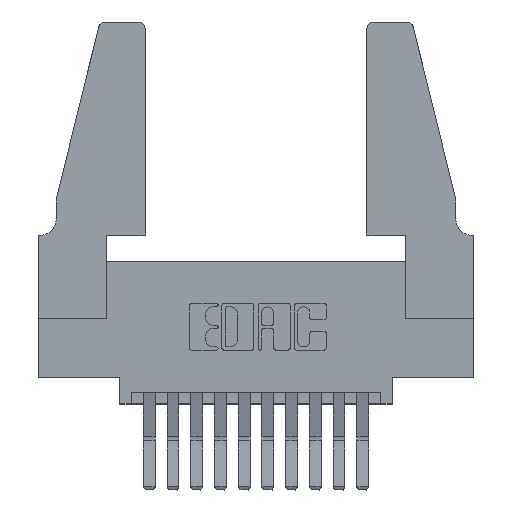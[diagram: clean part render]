
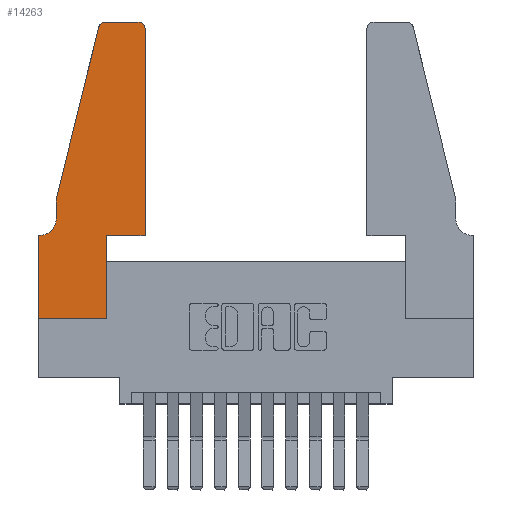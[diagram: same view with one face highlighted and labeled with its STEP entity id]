
A CAD part, top view. The second image highlights one B-rep face of the part: STEP entity #14263.
In plain terms, the highlighted planar face has unit normal (0, 0, 1).
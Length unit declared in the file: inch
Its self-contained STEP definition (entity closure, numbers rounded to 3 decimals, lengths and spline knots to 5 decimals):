
#20 = ORIENTED_EDGE ( 'NONE', *, *, #10793, .T. ) ;
#134 = VERTEX_POINT ( 'NONE', #2024 ) ;
#516 = CARTESIAN_POINT ( 'NONE',  ( 0.0755, 0.5, 0.37 ) ) ;
#620 = VERTEX_POINT ( 'NONE', #7448 ) ;
#683 = DIRECTION ( 'NONE',  ( 1., 0., 0. ) ) ;
#951 = CARTESIAN_POINT ( 'NONE',  ( 0.0755, 0.5, 0.37 ) ) ;
#965 = CARTESIAN_POINT ( 'NONE',  ( 0.4205, 1.22, 0.37 ) ) ;
#1316 = CARTESIAN_POINT ( 'NONE',  ( 0.0755, 0.5, 0.37 ) ) ;
#1519 = CARTESIAN_POINT ( 'NONE',  ( 0.2865, 0.35, 0.37 ) ) ;
#1893 = ORIENTED_EDGE ( 'NONE', *, *, #11716, .T. ) ;
#1920 = VECTOR ( 'NONE', #12752, 39.37008 ) ;
#2024 = CARTESIAN_POINT ( 'NONE',  ( 0., 0.35, 0.37 ) ) ;
#2279 = LINE ( 'NONE', #14541, #7880 ) ;
#2289 = DIRECTION ( 'NONE',  ( 1., 0., 0. ) ) ;
#2481 = CARTESIAN_POINT ( 'NONE',  ( 0.4205, 1.25, 0.37 ) ) ;
#2592 = DIRECTION ( 'NONE',  ( 0., -1., 0. ) ) ;
#2875 = EDGE_CURVE ( 'NONE', #134, #13438, #4953, .T. ) ;
#2930 = CIRCLE ( 'NONE', #3159, 0.03 ) ;
#3159 = AXIS2_PLACEMENT_3D ( 'NONE', #14060, #7624, #683 ) ;
#3321 = DIRECTION ( 'NONE',  ( 1., 0., 0. ) ) ;
#3361 = VERTEX_POINT ( 'NONE', #516 ) ;
#3426 = ORIENTED_EDGE ( 'NONE', *, *, #2875, .T. ) ;
#3492 = VECTOR ( 'NONE', #9399, 39.37008 ) ;
#3600 = VECTOR ( 'NONE', #2592, 39.37008 ) ;
#3761 = CARTESIAN_POINT ( 'NONE',  ( 0.4505, 0.35, 0.37 ) ) ;
#3775 = EDGE_CURVE ( 'NONE', #9336, #134, #2279, .T. ) ;
#3909 = CARTESIAN_POINT ( 'NONE',  ( 0.284, 1.25, 0.37 ) ) ;
#3928 = DIRECTION ( 'NONE',  ( -1., 0., 0. ) ) ;
#4141 = EDGE_CURVE ( 'NONE', #9167, #12550, #11786, .T. ) ;
#4200 = CARTESIAN_POINT ( 'NONE',  ( 0.4505, 1.22, 0.37 ) ) ;
#4295 = VECTOR ( 'NONE', #12698, 39.37008 ) ;
#4298 = EDGE_LOOP ( 'NONE', ( #11027, #5619, #14450, #20, #6785, #9504, #3426, #1893, #11402, #11693, #12188, #13279 ) ) ;
#4350 = VERTEX_POINT ( 'NONE', #4902 ) ;
#4546 = LINE ( 'NONE', #14178, #10050 ) ;
#4716 = EDGE_CURVE ( 'NONE', #6889, #4350, #4546, .T. ) ;
#4836 = DIRECTION ( 'NONE',  ( 0., 1., 0. ) ) ;
#4902 = CARTESIAN_POINT ( 'NONE',  ( 0.4505, 0.35, 0.37 ) ) ;
#4953 = LINE ( 'NONE', #8320, #1920 ) ;
#4991 = EDGE_CURVE ( 'NONE', #4350, #9167, #13086, .T. ) ;
#5003 = FACE_OUTER_BOUND ( 'NONE', #4298, .T. ) ;
#5048 = CARTESIAN_POINT ( 'NONE',  ( 0.2605, 1.25, 0.37 ) ) ;
#5599 = DIRECTION ( 'NONE',  ( -0.239, -0.971, 0. ) ) ;
#5619 = ORIENTED_EDGE ( 'NONE', *, *, #12937, .T. ) ;
#5859 = AXIS2_PLACEMENT_3D ( 'NONE', #965, #8966, #2289 ) ;
#6096 = DIRECTION ( 'NONE',  ( 0., 0., -1. ) ) ;
#6759 = AXIS2_PLACEMENT_3D ( 'NONE', #12670, #6096, #13705 ) ;
#6785 = ORIENTED_EDGE ( 'NONE', *, *, #11508, .T. ) ;
#6889 = VERTEX_POINT ( 'NONE', #13394 ) ;
#7047 = CARTESIAN_POINT ( 'NONE',  ( 0.25487, 1.22718, 0.37 ) ) ;
#7448 = CARTESIAN_POINT ( 'NONE',  ( 0.0755, 0.42, 0.37 ) ) ;
#7624 = DIRECTION ( 'NONE',  ( 0., 0., 1. ) ) ;
#7803 = VECTOR ( 'NONE', #5599, 39.37008 ) ;
#7880 = VECTOR ( 'NONE', #3928, 39.37008 ) ;
#8271 = CIRCLE ( 'NONE', #6759, 0.07 ) ;
#8320 = CARTESIAN_POINT ( 'NONE',  ( 0., 0., 0.37 ) ) ;
#8389 = EDGE_CURVE ( 'NONE', #8887, #6889, #9370, .T. ) ;
#8843 = PLANE ( 'NONE',  #11649 ) ;
#8887 = VERTEX_POINT ( 'NONE', #13555 ) ;
#8966 = DIRECTION ( 'NONE',  ( 0., 0., 1. ) ) ;
#8980 = VERTEX_POINT ( 'NONE', #3909 ) ;
#9167 = VERTEX_POINT ( 'NONE', #4200 ) ;
#9336 = VERTEX_POINT ( 'NONE', #13273 ) ;
#9370 = LINE ( 'NONE', #1519, #3492 ) ;
#9399 = DIRECTION ( 'NONE',  ( 0., 1., 0. ) ) ;
#9504 = ORIENTED_EDGE ( 'NONE', *, *, #3775, .T. ) ;
#9874 = CARTESIAN_POINT ( 'NONE',  ( 0., 0., 0.37 ) ) ;
#9928 = DIRECTION ( 'NONE',  ( 0., 0., 1. ) ) ;
#10050 = VECTOR ( 'NONE', #13141, 39.37008 ) ;
#10300 = EDGE_CURVE ( 'NONE', #12550, #8980, #12696, .T. ) ;
#10358 = LINE ( 'NONE', #951, #7803 ) ;
#10793 = EDGE_CURVE ( 'NONE', #3361, #620, #12368, .T. ) ;
#10971 = CARTESIAN_POINT ( 'NONE',  ( 0., 0.35, 0.37 ) ) ;
#11027 = ORIENTED_EDGE ( 'NONE', *, *, #10300, .T. ) ;
#11297 = VECTOR ( 'NONE', #13169, 39.37008 ) ;
#11402 = ORIENTED_EDGE ( 'NONE', *, *, #8389, .T. ) ;
#11439 = VERTEX_POINT ( 'NONE', #7047 ) ;
#11508 = EDGE_CURVE ( 'NONE', #620, #9336, #8271, .T. ) ;
#11649 = AXIS2_PLACEMENT_3D ( 'NONE', #10971, #9928, #3321 ) ;
#11693 = ORIENTED_EDGE ( 'NONE', *, *, #4716, .T. ) ;
#11716 = EDGE_CURVE ( 'NONE', #13438, #8887, #14117, .T. ) ;
#11786 = CIRCLE ( 'NONE', #5859, 0.03 ) ;
#12096 = VECTOR ( 'NONE', #4836, 39.37008 ) ;
#12188 = ORIENTED_EDGE ( 'NONE', *, *, #4991, .T. ) ;
#12368 = LINE ( 'NONE', #1316, #3600 ) ;
#12550 = VERTEX_POINT ( 'NONE', #2481 ) ;
#12670 = CARTESIAN_POINT ( 'NONE',  ( 0.0055, 0.42, 0.37 ) ) ;
#12696 = LINE ( 'NONE', #5048, #4295 ) ;
#12698 = DIRECTION ( 'NONE',  ( -1., 0., 0. ) ) ;
#12752 = DIRECTION ( 'NONE',  ( 0., -1., 0. ) ) ;
#12937 = EDGE_CURVE ( 'NONE', #8980, #11439, #2930, .T. ) ;
#13086 = LINE ( 'NONE', #3761, #12096 ) ;
#13141 = DIRECTION ( 'NONE',  ( 1., 0., 0. ) ) ;
#13169 = DIRECTION ( 'NONE',  ( 1., 0., 0. ) ) ;
#13273 = CARTESIAN_POINT ( 'NONE',  ( 0.0055, 0.35, 0.37 ) ) ;
#13279 = ORIENTED_EDGE ( 'NONE', *, *, #4141, .T. ) ;
#13394 = CARTESIAN_POINT ( 'NONE',  ( 0.2865, 0.35, 0.37 ) ) ;
#13438 = VERTEX_POINT ( 'NONE', #13914 ) ;
#13555 = CARTESIAN_POINT ( 'NONE',  ( 0.2865, 0., 0.37 ) ) ;
#13669 = EDGE_CURVE ( 'NONE', #11439, #3361, #10358, .T. ) ;
#13705 = DIRECTION ( 'NONE',  ( -1., 0., 0. ) ) ;
#13914 = CARTESIAN_POINT ( 'NONE',  ( 0., 0., 0.37 ) ) ;
#14060 = CARTESIAN_POINT ( 'NONE',  ( 0.284, 1.22, 0.37 ) ) ;
#14117 = LINE ( 'NONE', #9874, #11297 ) ;
#14178 = CARTESIAN_POINT ( 'NONE',  ( 0.4505, 0.35, 0.37 ) ) ;
#14263 = ADVANCED_FACE ( 'NONE', ( #5003 ), #8843, .T. ) ;
#14450 = ORIENTED_EDGE ( 'NONE', *, *, #13669, .T. ) ;
#14541 = CARTESIAN_POINT ( 'NONE',  ( 0.0755, 0.35, 0.37 ) ) ;
